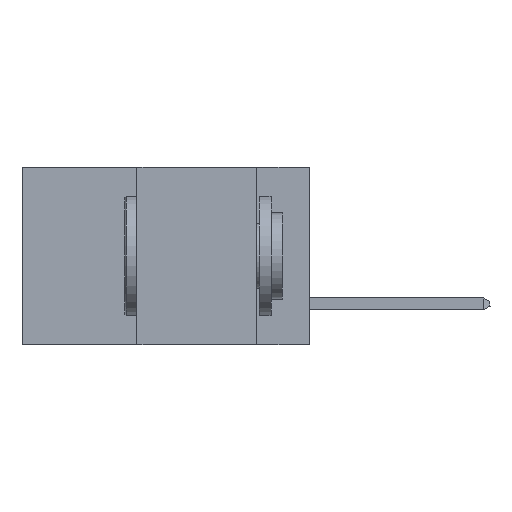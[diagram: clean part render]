
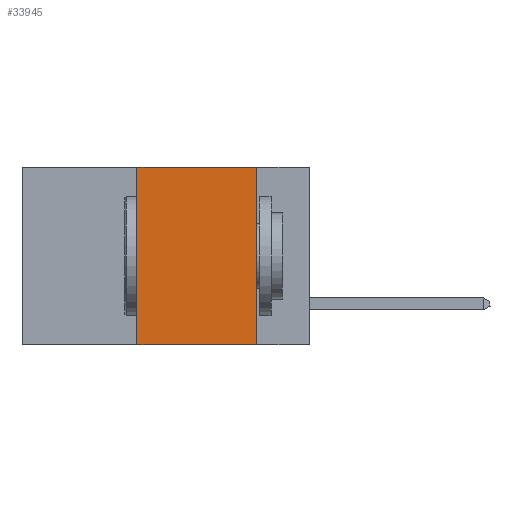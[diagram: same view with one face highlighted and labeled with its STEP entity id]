
A CAD part, left-side view. The second image highlights one B-rep face of the part: STEP entity #33945.
In plain terms, the highlighted planar face has unit normal (-1, 0, 0).
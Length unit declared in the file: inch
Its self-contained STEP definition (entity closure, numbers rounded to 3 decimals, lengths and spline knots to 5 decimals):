
#598 = FACE_OUTER_BOUND ( 'NONE', #35988, .T. ) ;
#1342 = EDGE_CURVE ( 'NONE', #4290, #7111, #14825, .T. ) ;
#2666 = EDGE_CURVE ( 'NONE', #22324, #35106, #13807, .T. ) ;
#4265 = CARTESIAN_POINT ( 'NONE',  ( 0., 0.11, 0. ) ) ;
#4290 = VERTEX_POINT ( 'NONE', #6252 ) ;
#5945 = VECTOR ( 'NONE', #23567, 39.37008 ) ;
#6120 = CARTESIAN_POINT ( 'NONE',  ( 0., 0.36, 0. ) ) ;
#6252 = CARTESIAN_POINT ( 'NONE',  ( 0., 0.36, -0.37 ) ) ;
#7111 = VERTEX_POINT ( 'NONE', #11608 ) ;
#9810 = EDGE_CURVE ( 'NONE', #7111, #22324, #24516, .T. ) ;
#11608 = CARTESIAN_POINT ( 'NONE',  ( 0., 0.36, 0. ) ) ;
#13082 = DIRECTION ( 'NONE',  ( 0., -1., 0. ) ) ;
#13807 = LINE ( 'NONE', #4265, #5945 ) ;
#14825 = LINE ( 'NONE', #6120, #17471 ) ;
#15791 = CARTESIAN_POINT ( 'NONE',  ( 0., 0.6, 0. ) ) ;
#16044 = CARTESIAN_POINT ( 'NONE',  ( 0., 0.6, 0. ) ) ;
#17471 = VECTOR ( 'NONE', #34118, 39.37008 ) ;
#19153 = AXIS2_PLACEMENT_3D ( 'NONE', #16044, #35481, #30119 ) ;
#21456 = ORIENTED_EDGE ( 'NONE', *, *, #9810, .F. ) ;
#22324 = VERTEX_POINT ( 'NONE', #26325 ) ;
#22856 = ORIENTED_EDGE ( 'NONE', *, *, #2666, .F. ) ;
#23567 = DIRECTION ( 'NONE',  ( 0., 0., -1. ) ) ;
#23934 = DIRECTION ( 'NONE',  ( 0., -1., 0. ) ) ;
#24422 = PLANE ( 'NONE',  #19153 ) ;
#24516 = LINE ( 'NONE', #15791, #33182 ) ;
#26007 = ORIENTED_EDGE ( 'NONE', *, *, #29849, .T. ) ;
#26325 = CARTESIAN_POINT ( 'NONE',  ( 0., 0.11, 0. ) ) ;
#26495 = ORIENTED_EDGE ( 'NONE', *, *, #1342, .F. ) ;
#27564 = VECTOR ( 'NONE', #13082, 39.37008 ) ;
#29849 = EDGE_CURVE ( 'NONE', #4290, #35106, #34523, .T. ) ;
#30119 = DIRECTION ( 'NONE',  ( 0., 0., -1. ) ) ;
#33133 = CARTESIAN_POINT ( 'NONE',  ( 0., 0.11, -0.37 ) ) ;
#33182 = VECTOR ( 'NONE', #23934, 39.37008 ) ;
#33945 = ADVANCED_FACE ( 'NONE', ( #598 ), #24422, .F. ) ;
#34118 = DIRECTION ( 'NONE',  ( 0., 0., 1. ) ) ;
#34523 = LINE ( 'NONE', #35569, #27564 ) ;
#35106 = VERTEX_POINT ( 'NONE', #33133 ) ;
#35481 = DIRECTION ( 'NONE',  ( 1., 0., 0. ) ) ;
#35569 = CARTESIAN_POINT ( 'NONE',  ( 0., 0.6, -0.37 ) ) ;
#35988 = EDGE_LOOP ( 'NONE', ( #22856, #21456, #26495, #26007 ) ) ;
